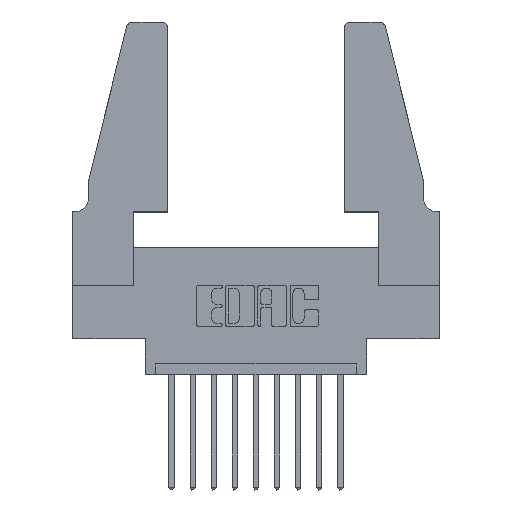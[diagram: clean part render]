
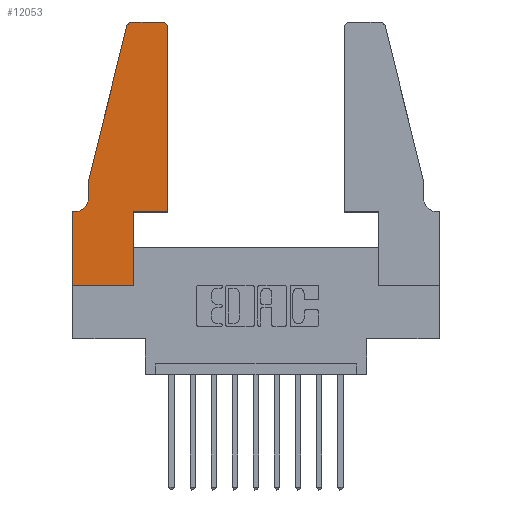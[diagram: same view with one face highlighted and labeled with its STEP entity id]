
A CAD part, top view. The second image highlights one B-rep face of the part: STEP entity #12053.
In plain terms, the highlighted planar face has unit normal (0, 0, 1).
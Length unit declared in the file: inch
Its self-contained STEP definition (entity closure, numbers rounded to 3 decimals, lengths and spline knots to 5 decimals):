
#91 = VERTEX_POINT ( 'NONE', #10295 ) ;
#106 = EDGE_CURVE ( 'NONE', #3646, #9648, #5711, .T. ) ;
#427 = CARTESIAN_POINT ( 'NONE',  ( 0.2605, 1.25, 0.37 ) ) ;
#592 = CARTESIAN_POINT ( 'NONE',  ( 0.4505, 0.35, 0.37 ) ) ;
#733 = DIRECTION ( 'NONE',  ( -1., 0., 0. ) ) ;
#1027 = CIRCLE ( 'NONE', #7106, 0.03 ) ;
#1057 = DIRECTION ( 'NONE',  ( 0., 0., 1. ) ) ;
#1192 = ORIENTED_EDGE ( 'NONE', *, *, #3879, .T. ) ;
#1277 = DIRECTION ( 'NONE',  ( 0., 0., 1. ) ) ;
#1660 = EDGE_CURVE ( 'NONE', #12352, #2198, #2562, .T. ) ;
#1662 = ORIENTED_EDGE ( 'NONE', *, *, #3279, .T. ) ;
#1678 = CIRCLE ( 'NONE', #13387, 0.07 ) ;
#1953 = ORIENTED_EDGE ( 'NONE', *, *, #1660, .T. ) ;
#2195 = AXIS2_PLACEMENT_3D ( 'NONE', #2919, #10242, #11218 ) ;
#2198 = VERTEX_POINT ( 'NONE', #2653 ) ;
#2220 = DIRECTION ( 'NONE',  ( 1., 0., 0. ) ) ;
#2373 = ORIENTED_EDGE ( 'NONE', *, *, #3268, .T. ) ;
#2385 = DIRECTION ( 'NONE',  ( 1., 0., 0. ) ) ;
#2562 = LINE ( 'NONE', #3878, #8928 ) ;
#2621 = ORIENTED_EDGE ( 'NONE', *, *, #106, .T. ) ;
#2630 = LINE ( 'NONE', #427, #5754 ) ;
#2653 = CARTESIAN_POINT ( 'NONE',  ( 0.0755, 0.5, 0.37 ) ) ;
#2919 = CARTESIAN_POINT ( 'NONE',  ( 0.284, 1.22, 0.37 ) ) ;
#2978 = VECTOR ( 'NONE', #2220, 39.37008 ) ;
#2993 = CARTESIAN_POINT ( 'NONE',  ( 0.2865, 0.35, 0.37 ) ) ;
#3210 = DIRECTION ( 'NONE',  ( 0., 0., -1. ) ) ;
#3268 = EDGE_CURVE ( 'NONE', #91, #12867, #1027, .T. ) ;
#3279 = EDGE_CURVE ( 'NONE', #4766, #11761, #1678, .T. ) ;
#3294 = LINE ( 'NONE', #11556, #2978 ) ;
#3358 = EDGE_CURVE ( 'NONE', #9648, #12236, #8048, .T. ) ;
#3646 = VERTEX_POINT ( 'NONE', #10038 ) ;
#3878 = CARTESIAN_POINT ( 'NONE',  ( 0.0755, 0.5, 0.37 ) ) ;
#3879 = EDGE_CURVE ( 'NONE', #7532, #12352, #11976, .T. ) ;
#4164 = LINE ( 'NONE', #10514, #5959 ) ;
#4313 = VECTOR ( 'NONE', #11418, 39.37008 ) ;
#4676 = ORIENTED_EDGE ( 'NONE', *, *, #10185, .T. ) ;
#4766 = VERTEX_POINT ( 'NONE', #13441 ) ;
#5078 = VECTOR ( 'NONE', #13310, 39.37008 ) ;
#5400 = CARTESIAN_POINT ( 'NONE',  ( 0.4205, 1.22, 0.37 ) ) ;
#5711 = LINE ( 'NONE', #8306, #8962 ) ;
#5754 = VECTOR ( 'NONE', #733, 39.37008 ) ;
#5791 = CARTESIAN_POINT ( 'NONE',  ( 0.2865, 0., 0.37 ) ) ;
#5875 = LINE ( 'NONE', #12714, #5078 ) ;
#5959 = VECTOR ( 'NONE', #6436, 39.37008 ) ;
#6069 = CARTESIAN_POINT ( 'NONE',  ( 0.25487, 1.22718, 0.37 ) ) ;
#6184 = AXIS2_PLACEMENT_3D ( 'NONE', #9469, #1277, #10532 ) ;
#6197 = VERTEX_POINT ( 'NONE', #7620 ) ;
#6346 = DIRECTION ( 'NONE',  ( -1., 0., 0. ) ) ;
#6436 = DIRECTION ( 'NONE',  ( -1., 0., 0. ) ) ;
#6574 = VECTOR ( 'NONE', #8828, 39.37008 ) ;
#6848 = VECTOR ( 'NONE', #11081, 39.37008 ) ;
#6998 = CARTESIAN_POINT ( 'NONE',  ( 0.0055, 0.35, 0.37 ) ) ;
#7106 = AXIS2_PLACEMENT_3D ( 'NONE', #5400, #1057, #7467 ) ;
#7282 = CARTESIAN_POINT ( 'NONE',  ( 0.284, 1.25, 0.37 ) ) ;
#7467 = DIRECTION ( 'NONE',  ( 1., 0., 0. ) ) ;
#7532 = VERTEX_POINT ( 'NONE', #7282 ) ;
#7620 = CARTESIAN_POINT ( 'NONE',  ( 0., 0.35, 0.37 ) ) ;
#7662 = EDGE_CURVE ( 'NONE', #11761, #6197, #4164, .T. ) ;
#8048 = LINE ( 'NONE', #2993, #4313 ) ;
#8306 = CARTESIAN_POINT ( 'NONE',  ( 0., 0., 0.37 ) ) ;
#8489 = PLANE ( 'NONE',  #6184 ) ;
#8569 = ORIENTED_EDGE ( 'NONE', *, *, #7662, .T. ) ;
#8712 = CARTESIAN_POINT ( 'NONE',  ( 0.4205, 1.25, 0.37 ) ) ;
#8761 = ORIENTED_EDGE ( 'NONE', *, *, #3358, .T. ) ;
#8828 = DIRECTION ( 'NONE',  ( 0., -1., 0. ) ) ;
#8928 = VECTOR ( 'NONE', #11315, 39.37008 ) ;
#8962 = VECTOR ( 'NONE', #2385, 39.37008 ) ;
#9115 = FACE_OUTER_BOUND ( 'NONE', #13057, .T. ) ;
#9377 = EDGE_CURVE ( 'NONE', #12236, #9715, #3294, .T. ) ;
#9469 = CARTESIAN_POINT ( 'NONE',  ( 0., 0.35, 0.37 ) ) ;
#9487 = CARTESIAN_POINT ( 'NONE',  ( 0.0055, 0.42, 0.37 ) ) ;
#9539 = ORIENTED_EDGE ( 'NONE', *, *, #9377, .T. ) ;
#9648 = VERTEX_POINT ( 'NONE', #5791 ) ;
#9715 = VERTEX_POINT ( 'NONE', #13338 ) ;
#10038 = CARTESIAN_POINT ( 'NONE',  ( 0., 0., 0.37 ) ) ;
#10052 = CARTESIAN_POINT ( 'NONE',  ( 0.2865, 0.35, 0.37 ) ) ;
#10185 = EDGE_CURVE ( 'NONE', #2198, #4766, #12112, .T. ) ;
#10242 = DIRECTION ( 'NONE',  ( 0., 0., 1. ) ) ;
#10295 = CARTESIAN_POINT ( 'NONE',  ( 0.4505, 1.22, 0.37 ) ) ;
#10514 = CARTESIAN_POINT ( 'NONE',  ( 0.0755, 0.35, 0.37 ) ) ;
#10532 = DIRECTION ( 'NONE',  ( 1., 0., 0. ) ) ;
#10724 = EDGE_CURVE ( 'NONE', #6197, #3646, #5875, .T. ) ;
#11081 = DIRECTION ( 'NONE',  ( 0., 1., 0. ) ) ;
#11218 = DIRECTION ( 'NONE',  ( 1., 0., 0. ) ) ;
#11315 = DIRECTION ( 'NONE',  ( -0.239, -0.971, 0. ) ) ;
#11395 = ORIENTED_EDGE ( 'NONE', *, *, #10724, .T. ) ;
#11418 = DIRECTION ( 'NONE',  ( 0., 1., 0. ) ) ;
#11556 = CARTESIAN_POINT ( 'NONE',  ( 0.4505, 0.35, 0.37 ) ) ;
#11698 = EDGE_CURVE ( 'NONE', #9715, #91, #12248, .T. ) ;
#11761 = VERTEX_POINT ( 'NONE', #6998 ) ;
#11791 = ORIENTED_EDGE ( 'NONE', *, *, #13514, .T. ) ;
#11936 = CARTESIAN_POINT ( 'NONE',  ( 0.0755, 0.5, 0.37 ) ) ;
#11976 = CIRCLE ( 'NONE', #2195, 0.03 ) ;
#12053 = ADVANCED_FACE ( 'NONE', ( #9115 ), #8489, .T. ) ;
#12112 = LINE ( 'NONE', #11936, #6574 ) ;
#12236 = VERTEX_POINT ( 'NONE', #10052 ) ;
#12248 = LINE ( 'NONE', #592, #6848 ) ;
#12352 = VERTEX_POINT ( 'NONE', #6069 ) ;
#12714 = CARTESIAN_POINT ( 'NONE',  ( 0., 0., 0.37 ) ) ;
#12867 = VERTEX_POINT ( 'NONE', #8712 ) ;
#13057 = EDGE_LOOP ( 'NONE', ( #11791, #1192, #1953, #4676, #1662, #8569, #11395, #2621, #8761, #9539, #13521, #2373 ) ) ;
#13310 = DIRECTION ( 'NONE',  ( 0., -1., 0. ) ) ;
#13338 = CARTESIAN_POINT ( 'NONE',  ( 0.4505, 0.35, 0.37 ) ) ;
#13387 = AXIS2_PLACEMENT_3D ( 'NONE', #9487, #3210, #6346 ) ;
#13441 = CARTESIAN_POINT ( 'NONE',  ( 0.0755, 0.42, 0.37 ) ) ;
#13514 = EDGE_CURVE ( 'NONE', #12867, #7532, #2630, .T. ) ;
#13521 = ORIENTED_EDGE ( 'NONE', *, *, #11698, .T. ) ;
